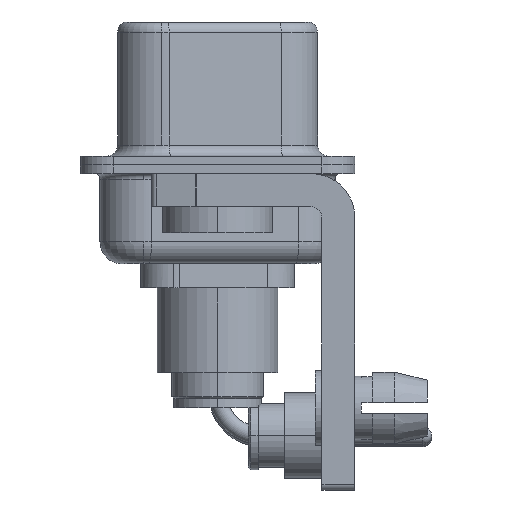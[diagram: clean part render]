
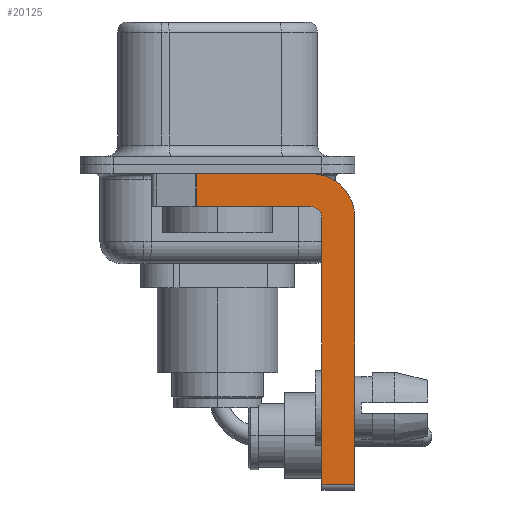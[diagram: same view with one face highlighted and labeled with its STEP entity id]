
A CAD part, left-side view. The second image highlights one B-rep face of the part: STEP entity #20125.
In plain terms, the highlighted planar face has unit normal (-1, 0, 0).
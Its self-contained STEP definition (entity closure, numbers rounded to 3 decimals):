
#40 = VERTEX_POINT ( 'NONE', #14935 ) ;
#105 = EDGE_LOOP ( 'NONE', ( #7977, #328, #8934, #6727, #18415, #11754, #19775, #21065 ) ) ;
#328 = ORIENTED_EDGE ( 'NONE', *, *, #10891, .T. ) ;
#448 = CARTESIAN_POINT ( 'NONE',  ( -2.9, -6.25, -2.4 ) ) ;
#693 = LINE ( 'NONE', #10808, #21840 ) ;
#893 = DIRECTION ( 'NONE',  ( -1., 0., 0. ) ) ;
#979 = DIRECTION ( 'NONE',  ( 0., 0., -1. ) ) ;
#1142 = CIRCLE ( 'NONE', #3672, 2. ) ;
#1209 = VECTOR ( 'NONE', #17713, 1000. ) ;
#1892 = CARTESIAN_POINT ( 'NONE',  ( -2.9, -4.25, -2.4 ) ) ;
#2251 = LINE ( 'NONE', #448, #1209 ) ;
#2361 = CARTESIAN_POINT ( 'NONE',  ( -2.9, 0.978, -1.9 ) ) ;
#2498 = DIRECTION ( 'NONE',  ( 0., -1., 0. ) ) ;
#2564 = CARTESIAN_POINT ( 'NONE',  ( -2.9, -4.25, -1.9 ) ) ;
#3672 = AXIS2_PLACEMENT_3D ( 'NONE', #18183, #9451, #11255 ) ;
#4737 = EDGE_CURVE ( 'NONE', #19259, #19627, #12920, .T. ) ;
#4911 = DIRECTION ( 'NONE',  ( 0., 0., 1. ) ) ;
#4957 = VERTEX_POINT ( 'NONE', #19373 ) ;
#5225 = DIRECTION ( 'NONE',  ( 0., -1., 0. ) ) ;
#5592 = AXIS2_PLACEMENT_3D ( 'NONE', #19759, #893, #17933 ) ;
#6727 = ORIENTED_EDGE ( 'NONE', *, *, #10383, .F. ) ;
#6887 = EDGE_CURVE ( 'NONE', #16359, #17470, #693, .T. ) ;
#7977 = ORIENTED_EDGE ( 'NONE', *, *, #6887, .F. ) ;
#7984 = CARTESIAN_POINT ( 'NONE',  ( -2.9, -4.75, -14.8 ) ) ;
#8146 = DIRECTION ( 'NONE',  ( 0., 1., 0. ) ) ;
#8499 = CIRCLE ( 'NONE', #5592, 0.5 ) ;
#8747 = CARTESIAN_POINT ( 'NONE',  ( -2.9, -4.25, -14.55 ) ) ;
#8934 = ORIENTED_EDGE ( 'NONE', *, *, #4737, .F. ) ;
#9251 = EDGE_CURVE ( 'NONE', #17227, #4957, #2251, .T. ) ;
#9451 = DIRECTION ( 'NONE',  ( 1., 0., 0. ) ) ;
#9815 = DIRECTION ( 'NONE',  ( 0., 0., -1. ) ) ;
#10383 = EDGE_CURVE ( 'NONE', #40, #19259, #8499, .T. ) ;
#10613 = CARTESIAN_POINT ( 'NONE',  ( -2.9, 0.978, -0.4 ) ) ;
#10808 = CARTESIAN_POINT ( 'NONE',  ( -2.9, 3., -0.4 ) ) ;
#10869 = FACE_OUTER_BOUND ( 'NONE', #105, .T. ) ;
#10891 = EDGE_CURVE ( 'NONE', #16359, #19627, #16297, .T. ) ;
#11255 = DIRECTION ( 'NONE',  ( 0., 0., -1. ) ) ;
#11360 = CARTESIAN_POINT ( 'NONE',  ( -2.9, -6.25, -2.4 ) ) ;
#11620 = LINE ( 'NONE', #7984, #20992 ) ;
#11754 = ORIENTED_EDGE ( 'NONE', *, *, #17382, .T. ) ;
#12920 = LINE ( 'NONE', #2564, #15974 ) ;
#14316 = VECTOR ( 'NONE', #9815, 1000. ) ;
#14919 = CARTESIAN_POINT ( 'NONE',  ( -2.9, 0.978, -1.9 ) ) ;
#14935 = CARTESIAN_POINT ( 'NONE',  ( -2.9, -4.75, -2.4 ) ) ;
#15302 = EDGE_CURVE ( 'NONE', #20994, #40, #11620, .T. ) ;
#15785 = LINE ( 'NONE', #8747, #15936 ) ;
#15936 = VECTOR ( 'NONE', #5225, 1000. ) ;
#15974 = VECTOR ( 'NONE', #8146, 1000. ) ;
#16297 = LINE ( 'NONE', #14919, #14316 ) ;
#16359 = VERTEX_POINT ( 'NONE', #10613 ) ;
#17227 = VERTEX_POINT ( 'NONE', #11360 ) ;
#17313 = PLANE ( 'NONE',  #18216 ) ;
#17382 = EDGE_CURVE ( 'NONE', #20994, #4957, #15785, .T. ) ;
#17470 = VERTEX_POINT ( 'NONE', #22369 ) ;
#17713 = DIRECTION ( 'NONE',  ( 0., 0., -1. ) ) ;
#17933 = DIRECTION ( 'NONE',  ( 0., 0., 1. ) ) ;
#18183 = CARTESIAN_POINT ( 'NONE',  ( -2.9, -4.25, -2.4 ) ) ;
#18216 = AXIS2_PLACEMENT_3D ( 'NONE', #1892, #21310, #979 ) ;
#18415 = ORIENTED_EDGE ( 'NONE', *, *, #15302, .F. ) ;
#19233 = EDGE_CURVE ( 'NONE', #17470, #17227, #1142, .T. ) ;
#19259 = VERTEX_POINT ( 'NONE', #21915 ) ;
#19373 = CARTESIAN_POINT ( 'NONE',  ( -2.9, -6.25, -14.55 ) ) ;
#19627 = VERTEX_POINT ( 'NONE', #2361 ) ;
#19759 = CARTESIAN_POINT ( 'NONE',  ( -2.9, -4.25, -2.4 ) ) ;
#19775 = ORIENTED_EDGE ( 'NONE', *, *, #9251, .F. ) ;
#20125 = ADVANCED_FACE ( 'NONE', ( #10869 ), #17313, .F. ) ;
#20734 = CARTESIAN_POINT ( 'NONE',  ( -2.9, -4.75, -14.55 ) ) ;
#20992 = VECTOR ( 'NONE', #4911, 1000. ) ;
#20994 = VERTEX_POINT ( 'NONE', #20734 ) ;
#21065 = ORIENTED_EDGE ( 'NONE', *, *, #19233, .F. ) ;
#21310 = DIRECTION ( 'NONE',  ( 1., 0., 0. ) ) ;
#21840 = VECTOR ( 'NONE', #2498, 1000. ) ;
#21915 = CARTESIAN_POINT ( 'NONE',  ( -2.9, -4.25, -1.9 ) ) ;
#22369 = CARTESIAN_POINT ( 'NONE',  ( -2.9, -4.25, -0.4 ) ) ;
